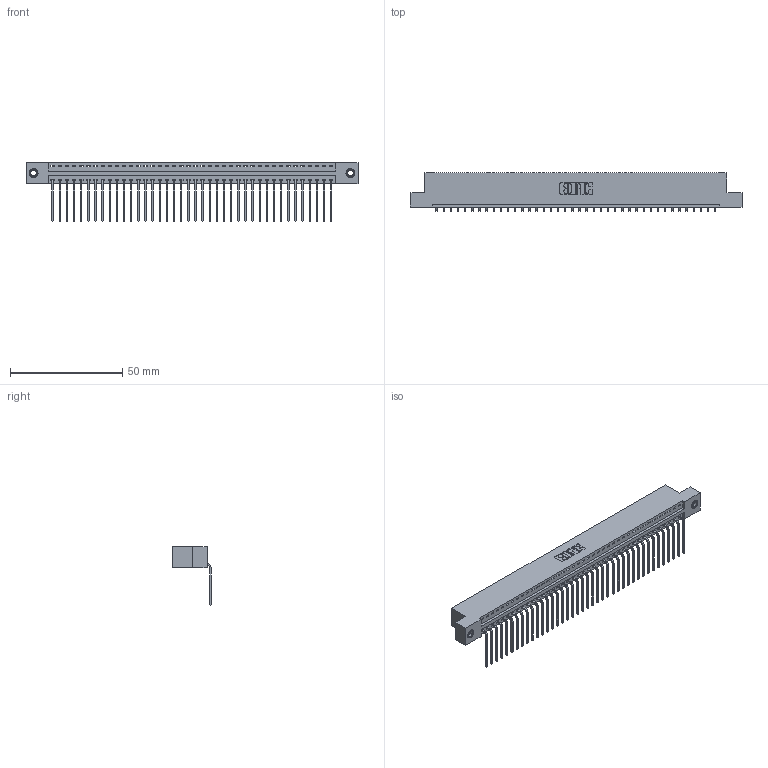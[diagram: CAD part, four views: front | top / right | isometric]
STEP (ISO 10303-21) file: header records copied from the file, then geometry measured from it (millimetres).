
FILE_DESCRIPTION (( 'STEP AP203' ), '1' );
FILE_NAME ('346-040-559-107.STEP', '2022-05-07T10:32:25', ( '' ), ( '' ), 'SwSTEP 2.0', 'SolidWorks 2020', '' );
FILE_SCHEMA (( 'CONFIG_CONTROL_DESIGN' ));
Length unit declared in the file: inch
Products named in the file (4): 345-250-001_345-250-005-103; 345-292-001_558 559 Tail - 1; 346 Part_Flush Mounting Lugs - 0.156 Dia-TI; 346-040-559-107
Assembly tree (43 placements, depth 2):
  346-040-559-107
    346 Part_Flush Mounting Lugs - 0.156 Dia-TI
    345-292-001_558 559 Tail - 1  x40
    345-250-001_345-250-005-103  x2
Bounding box: 147.57 x 17.08 x 26.16 mm (x, y, z)
Volume: 683.1 mm3; surface area: 18522.5 mm2
Topology: 42 solids, 43 shells, 2576 faces, 7744 edges, 5102 vertices
Faces by surface type: plane 1782, cylinder 778, cone 12, torus 4
Entity records: 26364 total; most frequent: CARTESIAN_POINT 4503, ORIENTED_EDGE 4470, DIRECTION 4001, EDGE_CURVE 2235, LINE 1923, VECTOR 1923, VERTEX_POINT 1484, AXIS2_PLACEMENT_3D 1039
